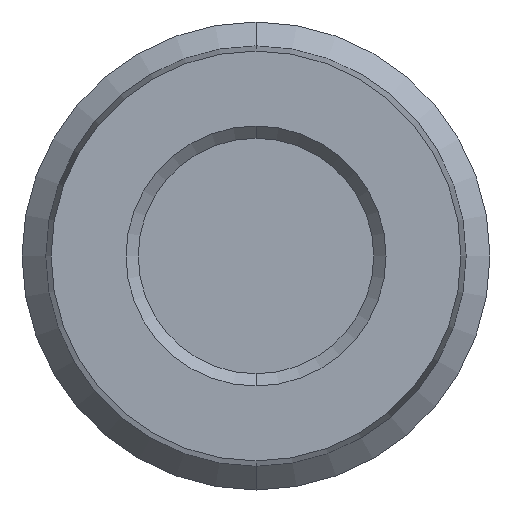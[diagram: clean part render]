
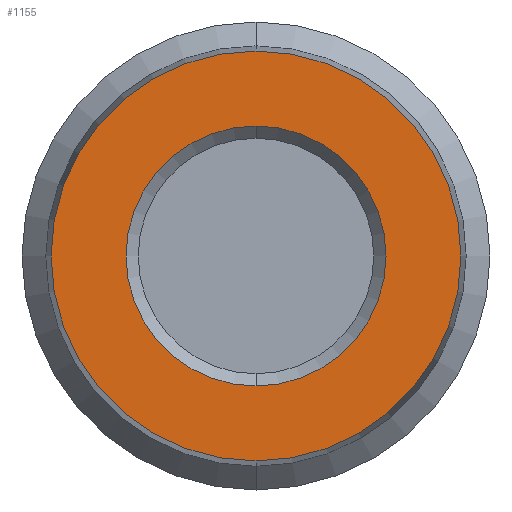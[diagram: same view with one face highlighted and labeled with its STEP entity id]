
A CAD part, front view. The second image highlights one B-rep face of the part: STEP entity #1155.
In plain terms, the highlighted planar face has unit normal (0, -1, 0).
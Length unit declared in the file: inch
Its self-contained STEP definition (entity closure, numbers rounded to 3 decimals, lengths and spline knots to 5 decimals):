
#16 = AXIS2_PLACEMENT_3D ( 'NONE', #1334, #1230, #401 ) ;
#26 = CARTESIAN_POINT ( 'NONE',  ( -4.56566, -1.00571, 2.03799 ) ) ;
#37 = AXIS2_PLACEMENT_3D ( 'NONE', #65, #482, #801 ) ;
#65 = CARTESIAN_POINT ( 'NONE',  ( -4.56566, -1.00571, 2.03799 ) ) ;
#111 = CIRCLE ( 'NONE', #1085, 0.67 ) ;
#138 = DIRECTION ( 'NONE',  ( 0., 0., -1. ) ) ;
#149 = VERTEX_POINT ( 'NONE', #1097 ) ;
#178 = FACE_OUTER_BOUND ( 'NONE', #617, .T. ) ;
#193 = ORIENTED_EDGE ( 'NONE', *, *, #1204, .T. ) ;
#233 = CIRCLE ( 'NONE', #37, 0.425 ) ;
#234 = EDGE_CURVE ( 'NONE', #149, #398, #1206, .T. ) ;
#263 = AXIS2_PLACEMENT_3D ( 'NONE', #708, #1037, #1129 ) ;
#290 = PLANE ( 'NONE',  #263 ) ;
#302 = AXIS2_PLACEMENT_3D ( 'NONE', #26, #645, #340 ) ;
#340 = DIRECTION ( 'NONE',  ( 0., 0., -1. ) ) ;
#397 = FACE_BOUND ( 'NONE', #546, .T. ) ;
#398 = VERTEX_POINT ( 'NONE', #1121 ) ;
#401 = DIRECTION ( 'NONE',  ( 0., 0., -1. ) ) ;
#449 = DIRECTION ( 'NONE',  ( 0., -1., 0. ) ) ;
#472 = ORIENTED_EDGE ( 'NONE', *, *, #548, .T. ) ;
#482 = DIRECTION ( 'NONE',  ( 0., -1., 0. ) ) ;
#546 = EDGE_LOOP ( 'NONE', ( #1060, #988 ) ) ;
#548 = EDGE_CURVE ( 'NONE', #1275, #710, #111, .T. ) ;
#614 = CIRCLE ( 'NONE', #16, 0.67 ) ;
#617 = EDGE_LOOP ( 'NONE', ( #193, #472 ) ) ;
#645 = DIRECTION ( 'NONE',  ( 0., -1., 0. ) ) ;
#708 = CARTESIAN_POINT ( 'NONE',  ( -4.56566, -1.00571, 0. ) ) ;
#710 = VERTEX_POINT ( 'NONE', #1363 ) ;
#801 = DIRECTION ( 'NONE',  ( 0., 0., -1. ) ) ;
#981 = CARTESIAN_POINT ( 'NONE',  ( -4.56566, -1.00571, 2.03799 ) ) ;
#988 = ORIENTED_EDGE ( 'NONE', *, *, #1324, .F. ) ;
#1037 = DIRECTION ( 'NONE',  ( 0., -1., 0. ) ) ;
#1060 = ORIENTED_EDGE ( 'NONE', *, *, #234, .F. ) ;
#1085 = AXIS2_PLACEMENT_3D ( 'NONE', #981, #449, #138 ) ;
#1097 = CARTESIAN_POINT ( 'NONE',  ( -4.56566, -1.00571, 1.61299 ) ) ;
#1121 = CARTESIAN_POINT ( 'NONE',  ( -4.56566, -1.00571, 2.46299 ) ) ;
#1129 = DIRECTION ( 'NONE',  ( 0., 0., -1. ) ) ;
#1133 = CARTESIAN_POINT ( 'NONE',  ( -4.56566, -1.00571, 1.36799 ) ) ;
#1155 = ADVANCED_FACE ( 'NONE', ( #397, #178 ), #290, .T. ) ;
#1204 = EDGE_CURVE ( 'NONE', #710, #1275, #614, .T. ) ;
#1206 = CIRCLE ( 'NONE', #302, 0.425 ) ;
#1230 = DIRECTION ( 'NONE',  ( 0., -1., 0. ) ) ;
#1275 = VERTEX_POINT ( 'NONE', #1133 ) ;
#1324 = EDGE_CURVE ( 'NONE', #398, #149, #233, .T. ) ;
#1334 = CARTESIAN_POINT ( 'NONE',  ( -4.56566, -1.00571, 2.03799 ) ) ;
#1363 = CARTESIAN_POINT ( 'NONE',  ( -4.56566, -1.00571, 2.70799 ) ) ;
